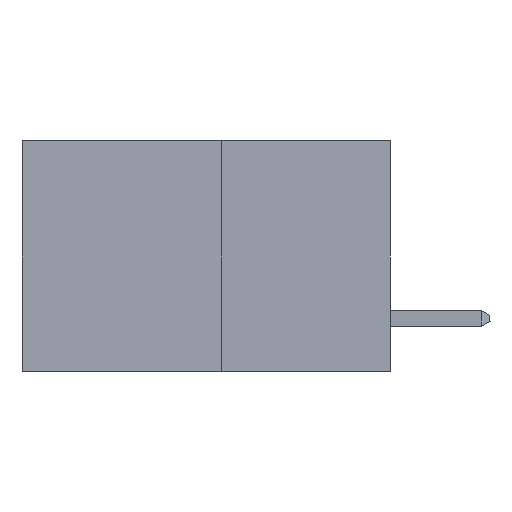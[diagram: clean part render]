
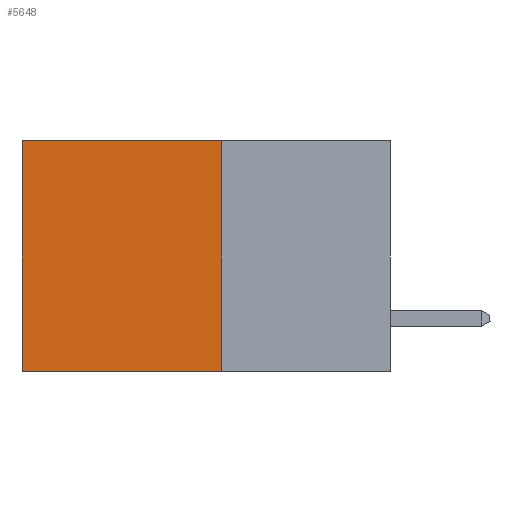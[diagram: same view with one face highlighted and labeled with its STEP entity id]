
A CAD part, left-side view. The second image highlights one B-rep face of the part: STEP entity #5648.
In plain terms, the highlighted planar face has unit normal (-1, 0, 0).
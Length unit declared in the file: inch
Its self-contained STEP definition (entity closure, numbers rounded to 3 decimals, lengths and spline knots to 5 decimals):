
#1756 = EDGE_CURVE ( 'NONE', #11722, #6895, #25349, .T. ) ;
#2208 = CARTESIAN_POINT ( 'NONE',  ( 0.277, 0.27, -0.37 ) ) ;
#2713 = VECTOR ( 'NONE', #22602, 39.37008 ) ;
#3482 = VERTEX_POINT ( 'NONE', #10401 ) ;
#4015 = FACE_OUTER_BOUND ( 'NONE', #31260, .T. ) ;
#4370 = DIRECTION ( 'NONE',  ( 0., 1., 0. ) ) ;
#5616 = EDGE_CURVE ( 'NONE', #14070, #6895, #12630, .T. ) ;
#5648 = ADVANCED_FACE ( 'NONE', ( #4015 ), #10129, .F. ) ;
#6784 = ORIENTED_EDGE ( 'NONE', *, *, #15182, .F. ) ;
#6895 = VERTEX_POINT ( 'NONE', #32774 ) ;
#10129 = PLANE ( 'NONE',  #32498 ) ;
#10401 = CARTESIAN_POINT ( 'NONE',  ( 0.277, 0.27, 0. ) ) ;
#11640 = VECTOR ( 'NONE', #22421, 39.37008 ) ;
#11722 = VERTEX_POINT ( 'NONE', #18903 ) ;
#12173 = CARTESIAN_POINT ( 'NONE',  ( 0.277, 0.27, 0. ) ) ;
#12630 = LINE ( 'NONE', #2208, #24741 ) ;
#14070 = VERTEX_POINT ( 'NONE', #23391 ) ;
#15182 = EDGE_CURVE ( 'NONE', #3482, #14070, #23446, .T. ) ;
#15323 = DIRECTION ( 'NONE',  ( 0., 0., -1. ) ) ;
#17042 = ORIENTED_EDGE ( 'NONE', *, *, #20535, .T. ) ;
#17509 = ORIENTED_EDGE ( 'NONE', *, *, #5616, .F. ) ;
#17632 = ORIENTED_EDGE ( 'NONE', *, *, #1756, .T. ) ;
#18903 = CARTESIAN_POINT ( 'NONE',  ( 0.277, 0.59, 0. ) ) ;
#20009 = CARTESIAN_POINT ( 'NONE',  ( 0.277, 0.27, -0.37 ) ) ;
#20535 = EDGE_CURVE ( 'NONE', #3482, #11722, #24286, .T. ) ;
#22421 = DIRECTION ( 'NONE',  ( 0., 0., -1. ) ) ;
#22602 = DIRECTION ( 'NONE',  ( 0., 0., -1. ) ) ;
#23391 = CARTESIAN_POINT ( 'NONE',  ( 0.277, 0.27, -0.37 ) ) ;
#23446 = LINE ( 'NONE', #20009, #2713 ) ;
#24286 = LINE ( 'NONE', #12173, #32166 ) ;
#24741 = VECTOR ( 'NONE', #33075, 39.37008 ) ;
#25349 = LINE ( 'NONE', #25987, #11640 ) ;
#25987 = CARTESIAN_POINT ( 'NONE',  ( 0.277, 0.59, -0.37 ) ) ;
#28117 = CARTESIAN_POINT ( 'NONE',  ( 0.277, 0.27, -0.37 ) ) ;
#30660 = DIRECTION ( 'NONE',  ( 1., 0., 0. ) ) ;
#31260 = EDGE_LOOP ( 'NONE', ( #17632, #17509, #6784, #17042 ) ) ;
#32166 = VECTOR ( 'NONE', #4370, 39.37008 ) ;
#32498 = AXIS2_PLACEMENT_3D ( 'NONE', #28117, #30660, #15323 ) ;
#32774 = CARTESIAN_POINT ( 'NONE',  ( 0.277, 0.59, -0.37 ) ) ;
#33075 = DIRECTION ( 'NONE',  ( 0., 1., 0. ) ) ;
